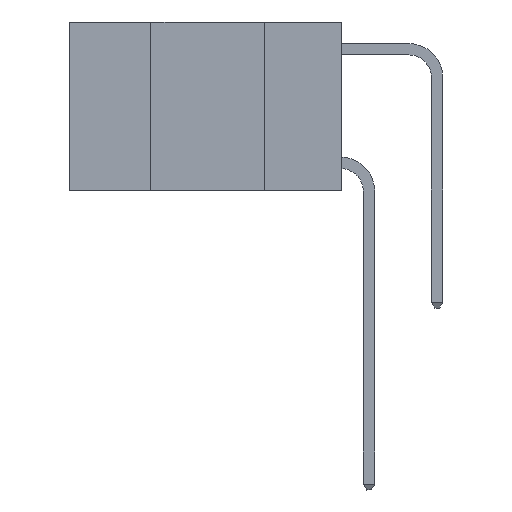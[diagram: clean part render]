
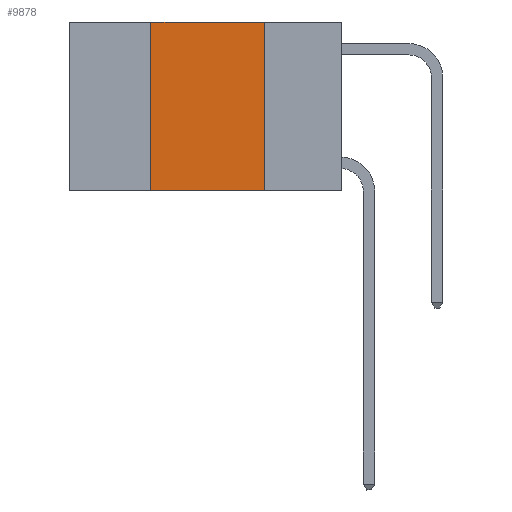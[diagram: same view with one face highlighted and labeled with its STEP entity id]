
A CAD part, left-side view. The second image highlights one B-rep face of the part: STEP entity #9878.
In plain terms, the highlighted planar face has unit normal (-1, 0, 0).
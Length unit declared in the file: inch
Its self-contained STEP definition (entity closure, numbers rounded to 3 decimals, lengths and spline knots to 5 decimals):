
#30 = VECTOR ( 'NONE', #6015, 39.37008 ) ;
#694 = DIRECTION ( 'NONE',  ( 0., 0., -1. ) ) ;
#774 = VERTEX_POINT ( 'NONE', #16050 ) ;
#1224 = DIRECTION ( 'NONE',  ( 1., 0., 0. ) ) ;
#1646 = CARTESIAN_POINT ( 'NONE',  ( 0., 0.42, 0. ) ) ;
#1774 = VERTEX_POINT ( 'NONE', #3647 ) ;
#2033 = VERTEX_POINT ( 'NONE', #18042 ) ;
#2818 = LINE ( 'NONE', #14023, #12366 ) ;
#3270 = ORIENTED_EDGE ( 'NONE', *, *, #6844, .F. ) ;
#3647 = CARTESIAN_POINT ( 'NONE',  ( 0., 0.17, 0. ) ) ;
#3780 = ORIENTED_EDGE ( 'NONE', *, *, #12403, .F. ) ;
#4359 = EDGE_CURVE ( 'NONE', #13201, #2033, #2818, .T. ) ;
#5290 = VECTOR ( 'NONE', #13139, 39.37008 ) ;
#5516 = DIRECTION ( 'NONE',  ( 0., 0., -1. ) ) ;
#6015 = DIRECTION ( 'NONE',  ( 0., -1., 0. ) ) ;
#6844 = EDGE_CURVE ( 'NONE', #13201, #774, #11457, .T. ) ;
#7717 = ORIENTED_EDGE ( 'NONE', *, *, #4359, .T. ) ;
#8128 = DIRECTION ( 'NONE',  ( 0., -1., 0. ) ) ;
#8595 = EDGE_LOOP ( 'NONE', ( #13562, #3780, #3270, #7717 ) ) ;
#9002 = LINE ( 'NONE', #10503, #30 ) ;
#9878 = ADVANCED_FACE ( 'NONE', ( #12419 ), #15430, .F. ) ;
#10503 = CARTESIAN_POINT ( 'NONE',  ( 0., 0.6, 0. ) ) ;
#10759 = VECTOR ( 'NONE', #694, 39.37008 ) ;
#11457 = LINE ( 'NONE', #1646, #5290 ) ;
#11992 = LINE ( 'NONE', #12082, #10759 ) ;
#12082 = CARTESIAN_POINT ( 'NONE',  ( 0., 0.17, 0. ) ) ;
#12366 = VECTOR ( 'NONE', #8128, 39.37008 ) ;
#12403 = EDGE_CURVE ( 'NONE', #774, #1774, #9002, .T. ) ;
#12419 = FACE_OUTER_BOUND ( 'NONE', #8595, .T. ) ;
#12554 = EDGE_CURVE ( 'NONE', #1774, #2033, #11992, .T. ) ;
#13139 = DIRECTION ( 'NONE',  ( 0., 0., 1. ) ) ;
#13201 = VERTEX_POINT ( 'NONE', #16091 ) ;
#13384 = AXIS2_PLACEMENT_3D ( 'NONE', #14014, #1224, #5516 ) ;
#13562 = ORIENTED_EDGE ( 'NONE', *, *, #12554, .F. ) ;
#14014 = CARTESIAN_POINT ( 'NONE',  ( 0., 0.6, 0. ) ) ;
#14023 = CARTESIAN_POINT ( 'NONE',  ( 0., 0.6, -0.37 ) ) ;
#15430 = PLANE ( 'NONE',  #13384 ) ;
#16050 = CARTESIAN_POINT ( 'NONE',  ( 0., 0.42, 0. ) ) ;
#16091 = CARTESIAN_POINT ( 'NONE',  ( 0., 0.42, -0.37 ) ) ;
#18042 = CARTESIAN_POINT ( 'NONE',  ( 0., 0.17, -0.37 ) ) ;
